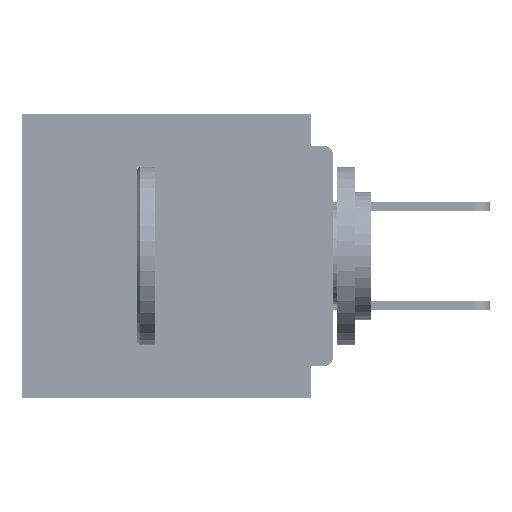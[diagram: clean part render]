
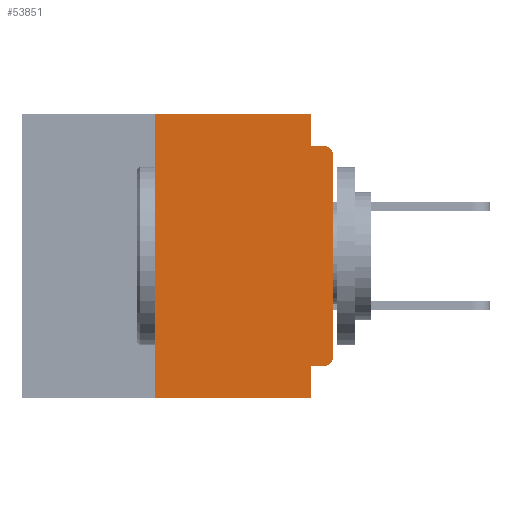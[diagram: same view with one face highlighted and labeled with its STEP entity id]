
A CAD part, left-side view. The second image highlights one B-rep face of the part: STEP entity #53851.
In plain terms, the highlighted planar face has unit normal (-1, 0, 0).
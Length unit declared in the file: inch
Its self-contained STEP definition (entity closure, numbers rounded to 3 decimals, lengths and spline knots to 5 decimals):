
#454 = CARTESIAN_POINT ( 'NONE',  ( 0., 0.015, -0.045 ) ) ;
#1121 = ORIENTED_EDGE ( 'NONE', *, *, #41712, .F. ) ;
#1521 = VECTOR ( 'NONE', #26278, 39.37008 ) ;
#2140 = EDGE_CURVE ( 'NONE', #62459, #14196, #40171, .T. ) ;
#2300 = FACE_OUTER_BOUND ( 'NONE', #31362, .T. ) ;
#4282 = ORIENTED_EDGE ( 'NONE', *, *, #52167, .T. ) ;
#4371 = ORIENTED_EDGE ( 'NONE', *, *, #2140, .F. ) ;
#5476 = CARTESIAN_POINT ( 'NONE',  ( 0., 0.031, 0. ) ) ;
#5580 = DIRECTION ( 'NONE',  ( -1., 0., 0. ) ) ;
#5746 = PLANE ( 'NONE',  #27145 ) ;
#7374 = DIRECTION ( 'NONE',  ( 0., -1., 0. ) ) ;
#7608 = LINE ( 'NONE', #56642, #31853 ) ;
#10391 = VECTOR ( 'NONE', #24236, 39.37008 ) ;
#10605 = DIRECTION ( 'NONE',  ( 0., 0., -1. ) ) ;
#14196 = VERTEX_POINT ( 'NONE', #30738 ) ;
#14703 = CARTESIAN_POINT ( 'NONE',  ( 0., 0., -0.355 ) ) ;
#15558 = DIRECTION ( 'NONE',  ( -1., 0., 0. ) ) ;
#15753 = EDGE_CURVE ( 'NONE', #40408, #30592, #55065, .T. ) ;
#15991 = CARTESIAN_POINT ( 'NONE',  ( 0., 0., 0. ) ) ;
#16868 = CARTESIAN_POINT ( 'NONE',  ( 0., 0.031, -0.4 ) ) ;
#17260 = ORIENTED_EDGE ( 'NONE', *, *, #37950, .T. ) ;
#17651 = CARTESIAN_POINT ( 'NONE',  ( 0., 0.031, -0.355 ) ) ;
#18710 = VERTEX_POINT ( 'NONE', #41124 ) ;
#20106 = CARTESIAN_POINT ( 'NONE',  ( 0., 0.437, 0. ) ) ;
#21620 = CARTESIAN_POINT ( 'NONE',  ( 0., 0.25, 0. ) ) ;
#23112 = VECTOR ( 'NONE', #24399, 39.37008 ) ;
#24040 = LINE ( 'NONE', #16868, #62620 ) ;
#24236 = DIRECTION ( 'NONE',  ( 0., -1., 0. ) ) ;
#24399 = DIRECTION ( 'NONE',  ( 0., 1., 0. ) ) ;
#26278 = DIRECTION ( 'NONE',  ( 0., 0., -1. ) ) ;
#27145 = AXIS2_PLACEMENT_3D ( 'NONE', #20106, #39589, #10605 ) ;
#28910 = VECTOR ( 'NONE', #36298, 39.37008 ) ;
#29099 = VERTEX_POINT ( 'NONE', #21620 ) ;
#29366 = VECTOR ( 'NONE', #54667, 39.37008 ) ;
#30592 = VERTEX_POINT ( 'NONE', #55521 ) ;
#30738 = CARTESIAN_POINT ( 'NONE',  ( 0., 0.031, -0.045 ) ) ;
#31362 = EDGE_LOOP ( 'NONE', ( #48982, #4282, #1121, #4371, #37860, #34067, #17260, #32724, #42725, #31715 ) ) ;
#31715 = ORIENTED_EDGE ( 'NONE', *, *, #36731, .T. ) ;
#31853 = VECTOR ( 'NONE', #61499, 39.37008 ) ;
#32724 = ORIENTED_EDGE ( 'NONE', *, *, #54698, .F. ) ;
#34067 = ORIENTED_EDGE ( 'NONE', *, *, #58986, .F. ) ;
#34363 = AXIS2_PLACEMENT_3D ( 'NONE', #44482, #15558, #49344 ) ;
#34567 = CARTESIAN_POINT ( 'NONE',  ( 0., 0.015, -0.34 ) ) ;
#34903 = VERTEX_POINT ( 'NONE', #37200 ) ;
#36100 = DIRECTION ( 'NONE',  ( 0., 0., -1. ) ) ;
#36298 = DIRECTION ( 'NONE',  ( 0., 0., 1. ) ) ;
#36624 = CIRCLE ( 'NONE', #34363, 0.015 ) ;
#36731 = EDGE_CURVE ( 'NONE', #18710, #40408, #51411, .T. ) ;
#37200 = CARTESIAN_POINT ( 'NONE',  ( 0., 0.25, -0.4 ) ) ;
#37860 = ORIENTED_EDGE ( 'NONE', *, *, #47958, .F. ) ;
#37950 = EDGE_CURVE ( 'NONE', #34903, #51832, #61813, .T. ) ;
#38908 = EDGE_CURVE ( 'NONE', #18710, #46926, #50377, .T. ) ;
#39435 = DIRECTION ( 'NONE',  ( 0., 0., -1. ) ) ;
#39589 = DIRECTION ( 'NONE',  ( 1., 0., 0. ) ) ;
#40171 = LINE ( 'NONE', #50365, #1521 ) ;
#40408 = VERTEX_POINT ( 'NONE', #40751 ) ;
#40751 = CARTESIAN_POINT ( 'NONE',  ( 0., 0., -0.34 ) ) ;
#41124 = CARTESIAN_POINT ( 'NONE',  ( 0., 0.015, -0.355 ) ) ;
#41712 = EDGE_CURVE ( 'NONE', #14196, #60987, #7608, .T. ) ;
#41762 = LINE ( 'NONE', #43326, #28910 ) ;
#42725 = ORIENTED_EDGE ( 'NONE', *, *, #38908, .F. ) ;
#43326 = CARTESIAN_POINT ( 'NONE',  ( 0., 0.25, -0.4 ) ) ;
#44102 = AXIS2_PLACEMENT_3D ( 'NONE', #34567, #5580, #39435 ) ;
#44482 = CARTESIAN_POINT ( 'NONE',  ( 0., 0.015, -0.06 ) ) ;
#46219 = VECTOR ( 'NONE', #7374, 39.37008 ) ;
#46926 = VERTEX_POINT ( 'NONE', #17651 ) ;
#47958 = EDGE_CURVE ( 'NONE', #29099, #62459, #59042, .T. ) ;
#48982 = ORIENTED_EDGE ( 'NONE', *, *, #15753, .T. ) ;
#49344 = DIRECTION ( 'NONE',  ( 0., 0., -1. ) ) ;
#50365 = CARTESIAN_POINT ( 'NONE',  ( 0., 0.031, 0. ) ) ;
#50377 = LINE ( 'NONE', #14703, #23112 ) ;
#51411 = CIRCLE ( 'NONE', #44102, 0.015 ) ;
#51832 = VERTEX_POINT ( 'NONE', #60162 ) ;
#52167 = EDGE_CURVE ( 'NONE', #30592, #60987, #36624, .T. ) ;
#53851 = ADVANCED_FACE ( 'NONE', ( #2300 ), #5746, .F. ) ;
#54667 = DIRECTION ( 'NONE',  ( 0., 0., 1. ) ) ;
#54698 = EDGE_CURVE ( 'NONE', #46926, #51832, #24040, .T. ) ;
#55065 = LINE ( 'NONE', #15991, #29366 ) ;
#55521 = CARTESIAN_POINT ( 'NONE',  ( 0., 0., -0.06 ) ) ;
#55593 = CARTESIAN_POINT ( 'NONE',  ( 0., 0.437, 0. ) ) ;
#56642 = CARTESIAN_POINT ( 'NONE',  ( 0., 0., -0.045 ) ) ;
#58061 = CARTESIAN_POINT ( 'NONE',  ( 0., 0.437, -0.4 ) ) ;
#58986 = EDGE_CURVE ( 'NONE', #34903, #29099, #41762, .T. ) ;
#59042 = LINE ( 'NONE', #55593, #46219 ) ;
#60162 = CARTESIAN_POINT ( 'NONE',  ( 0., 0.031, -0.4 ) ) ;
#60987 = VERTEX_POINT ( 'NONE', #454 ) ;
#61499 = DIRECTION ( 'NONE',  ( 0., -1., 0. ) ) ;
#61813 = LINE ( 'NONE', #58061, #10391 ) ;
#62459 = VERTEX_POINT ( 'NONE', #5476 ) ;
#62620 = VECTOR ( 'NONE', #36100, 39.37008 ) ;
